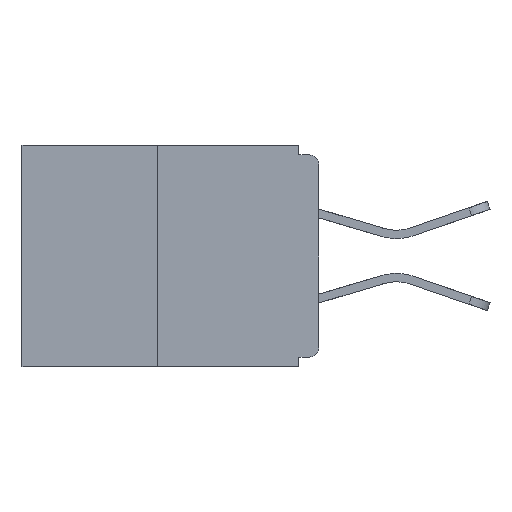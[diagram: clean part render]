
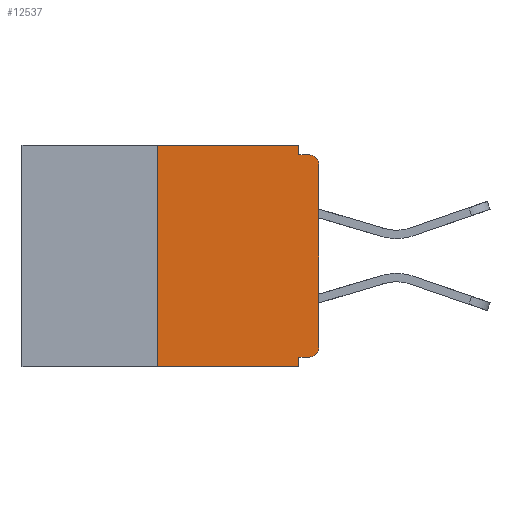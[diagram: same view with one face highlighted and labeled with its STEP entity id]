
A CAD part, left-side view. The second image highlights one B-rep face of the part: STEP entity #12537.
In plain terms, the highlighted planar face has unit normal (-1, 0, 0).
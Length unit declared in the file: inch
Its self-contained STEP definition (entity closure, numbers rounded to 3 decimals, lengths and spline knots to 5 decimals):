
#92 = VERTEX_POINT ( 'NONE', #4896 ) ;
#276 = VECTOR ( 'NONE', #3292, 39.37008 ) ;
#312 = VECTOR ( 'NONE', #7725, 39.37008 ) ;
#314 = VECTOR ( 'NONE', #14435, 39.37008 ) ;
#443 = EDGE_CURVE ( 'NONE', #1266, #7249, #971, .T. ) ;
#570 = CARTESIAN_POINT ( 'NONE',  ( 0., 0.031, 0. ) ) ;
#607 = VERTEX_POINT ( 'NONE', #6222 ) ;
#971 = CIRCLE ( 'NONE', #9852, 0.015 ) ;
#973 = ORIENTED_EDGE ( 'NONE', *, *, #12026, .F. ) ;
#1060 = DIRECTION ( 'NONE',  ( 0., 1., 0. ) ) ;
#1080 = VERTEX_POINT ( 'NONE', #570 ) ;
#1132 = ORIENTED_EDGE ( 'NONE', *, *, #8164, .F. ) ;
#1187 = CARTESIAN_POINT ( 'NONE',  ( 0., 0.031, 0. ) ) ;
#1208 = DIRECTION ( 'NONE',  ( -1., 0., 0. ) ) ;
#1266 = VERTEX_POINT ( 'NONE', #4406 ) ;
#1419 = DIRECTION ( 'NONE',  ( 0., -1., 0. ) ) ;
#1893 = VECTOR ( 'NONE', #1419, 39.37008 ) ;
#1998 = EDGE_CURVE ( 'NONE', #10274, #14738, #7238, .T. ) ;
#3192 = DIRECTION ( 'NONE',  ( 0., 0., -1. ) ) ;
#3292 = DIRECTION ( 'NONE',  ( 0., -1., 0. ) ) ;
#3664 = DIRECTION ( 'NONE',  ( 0., 0., -1. ) ) ;
#4335 = LINE ( 'NONE', #14751, #312 ) ;
#4402 = VERTEX_POINT ( 'NONE', #7954 ) ;
#4406 = CARTESIAN_POINT ( 'NONE',  ( 0., 0.015, -0.328 ) ) ;
#4597 = CIRCLE ( 'NONE', #12511, 0.015 ) ;
#4894 = ORIENTED_EDGE ( 'NONE', *, *, #1998, .F. ) ;
#4896 = CARTESIAN_POINT ( 'NONE',  ( 0., 0.031, -0.015 ) ) ;
#4939 = ORIENTED_EDGE ( 'NONE', *, *, #11762, .T. ) ;
#5027 = VECTOR ( 'NONE', #3664, 39.37008 ) ;
#5337 = LINE ( 'NONE', #8800, #6964 ) ;
#5364 = CARTESIAN_POINT ( 'NONE',  ( 0., 0.46, 0. ) ) ;
#5497 = LINE ( 'NONE', #6784, #6829 ) ;
#5545 = LINE ( 'NONE', #13481, #276 ) ;
#5720 = CARTESIAN_POINT ( 'NONE',  ( 0., 0.031, -0.328 ) ) ;
#5724 = DIRECTION ( 'NONE',  ( -1., 0., 0. ) ) ;
#5843 = EDGE_CURVE ( 'NONE', #9394, #4402, #6426, .T. ) ;
#5942 = CARTESIAN_POINT ( 'NONE',  ( 0., 0.015, -0.03 ) ) ;
#6181 = CARTESIAN_POINT ( 'NONE',  ( 0., 0.25, 0. ) ) ;
#6222 = CARTESIAN_POINT ( 'NONE',  ( 0., 0.015, -0.015 ) ) ;
#6265 = ORIENTED_EDGE ( 'NONE', *, *, #5843, .F. ) ;
#6426 = LINE ( 'NONE', #9887, #314 ) ;
#6494 = PLANE ( 'NONE',  #11571 ) ;
#6784 = CARTESIAN_POINT ( 'NONE',  ( 0., 0., -0.328 ) ) ;
#6807 = EDGE_CURVE ( 'NONE', #1266, #9394, #5497, .T. ) ;
#6829 = VECTOR ( 'NONE', #1060, 39.37008 ) ;
#6916 = LINE ( 'NONE', #1187, #5027 ) ;
#6937 = DIRECTION ( 'NONE',  ( 0., 0., -1. ) ) ;
#6964 = VECTOR ( 'NONE', #13363, 39.37008 ) ;
#7033 = ORIENTED_EDGE ( 'NONE', *, *, #6807, .F. ) ;
#7091 = CARTESIAN_POINT ( 'NONE',  ( 0., 0.25, 0. ) ) ;
#7238 = LINE ( 'NONE', #6181, #8494 ) ;
#7249 = VERTEX_POINT ( 'NONE', #10290 ) ;
#7416 = EDGE_CURVE ( 'NONE', #7249, #13905, #5337, .T. ) ;
#7725 = DIRECTION ( 'NONE',  ( 0., -1., 0. ) ) ;
#7776 = FACE_OUTER_BOUND ( 'NONE', #13608, .T. ) ;
#7844 = EDGE_CURVE ( 'NONE', #14738, #1080, #9682, .T. ) ;
#7954 = CARTESIAN_POINT ( 'NONE',  ( 0., 0.031, -0.343 ) ) ;
#8164 = EDGE_CURVE ( 'NONE', #1080, #92, #6916, .T. ) ;
#8264 = ORIENTED_EDGE ( 'NONE', *, *, #443, .T. ) ;
#8494 = VECTOR ( 'NONE', #10756, 39.37008 ) ;
#8800 = CARTESIAN_POINT ( 'NONE',  ( 0., 0., 0. ) ) ;
#9335 = CARTESIAN_POINT ( 'NONE',  ( 0., 0.015, -0.313 ) ) ;
#9394 = VERTEX_POINT ( 'NONE', #5720 ) ;
#9682 = LINE ( 'NONE', #12896, #1893 ) ;
#9852 = AXIS2_PLACEMENT_3D ( 'NONE', #9335, #1208, #6937 ) ;
#9887 = CARTESIAN_POINT ( 'NONE',  ( 0., 0.031, -0.343 ) ) ;
#9957 = DIRECTION ( 'NONE',  ( 1., 0., 0. ) ) ;
#10274 = VERTEX_POINT ( 'NONE', #14054 ) ;
#10290 = CARTESIAN_POINT ( 'NONE',  ( 0., 0., -0.313 ) ) ;
#10749 = ORIENTED_EDGE ( 'NONE', *, *, #7844, .F. ) ;
#10756 = DIRECTION ( 'NONE',  ( 0., 0., 1. ) ) ;
#10773 = CARTESIAN_POINT ( 'NONE',  ( 0., 0., -0.03 ) ) ;
#11571 = AXIS2_PLACEMENT_3D ( 'NONE', #5364, #9957, #3192 ) ;
#11614 = ORIENTED_EDGE ( 'NONE', *, *, #7416, .T. ) ;
#11762 = EDGE_CURVE ( 'NONE', #13905, #607, #4597, .T. ) ;
#12026 = EDGE_CURVE ( 'NONE', #92, #607, #5545, .T. ) ;
#12511 = AXIS2_PLACEMENT_3D ( 'NONE', #5942, #5724, #12535 ) ;
#12535 = DIRECTION ( 'NONE',  ( 0., 0., -1. ) ) ;
#12537 = ADVANCED_FACE ( 'NONE', ( #7776 ), #6494, .F. ) ;
#12896 = CARTESIAN_POINT ( 'NONE',  ( 0., 0.46, 0. ) ) ;
#13363 = DIRECTION ( 'NONE',  ( 0., 0., 1. ) ) ;
#13481 = CARTESIAN_POINT ( 'NONE',  ( 0., 0., -0.015 ) ) ;
#13608 = EDGE_LOOP ( 'NONE', ( #10749, #4894, #14735, #6265, #7033, #8264, #11614, #4939, #973, #1132 ) ) ;
#13609 = EDGE_CURVE ( 'NONE', #10274, #4402, #4335, .T. ) ;
#13905 = VERTEX_POINT ( 'NONE', #10773 ) ;
#14054 = CARTESIAN_POINT ( 'NONE',  ( 0., 0.25, -0.343 ) ) ;
#14435 = DIRECTION ( 'NONE',  ( 0., 0., -1. ) ) ;
#14735 = ORIENTED_EDGE ( 'NONE', *, *, #13609, .T. ) ;
#14738 = VERTEX_POINT ( 'NONE', #7091 ) ;
#14751 = CARTESIAN_POINT ( 'NONE',  ( 0., 0.46, -0.343 ) ) ;
